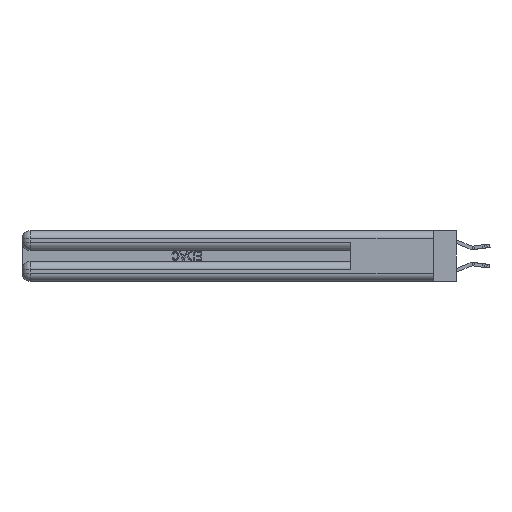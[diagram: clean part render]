
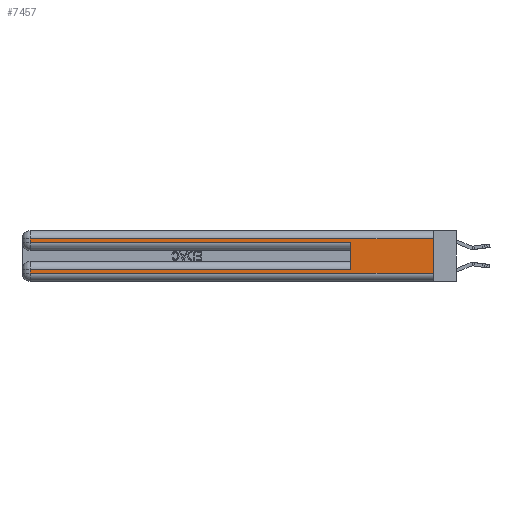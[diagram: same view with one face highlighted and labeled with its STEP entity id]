
A CAD part, left-side view. The second image highlights one B-rep face of the part: STEP entity #7457.
In plain terms, the highlighted planar face has unit normal (-1, 0, 0).
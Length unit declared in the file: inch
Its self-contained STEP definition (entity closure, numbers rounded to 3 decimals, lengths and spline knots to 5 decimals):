
#335 = CARTESIAN_POINT ( 'NONE',  ( 0., 0., 0.285 ) ) ;
#734 = VECTOR ( 'NONE', #7939, 39.37008 ) ;
#883 = DIRECTION ( 'NONE',  ( 0., 0., -1. ) ) ;
#1002 = LINE ( 'NONE', #26193, #14297 ) ;
#1200 = VERTEX_POINT ( 'NONE', #1347 ) ;
#1347 = CARTESIAN_POINT ( 'NONE',  ( 0., 0.6, 0.085 ) ) ;
#1394 = LINE ( 'NONE', #22031, #15465 ) ;
#2691 = DIRECTION ( 'NONE',  ( 0., 0., -1. ) ) ;
#3408 = EDGE_CURVE ( 'NONE', #15982, #7202, #14040, .T. ) ;
#3875 = ORIENTED_EDGE ( 'NONE', *, *, #21778, .F. ) ;
#4414 = DIRECTION ( 'NONE',  ( 0., 0., 1. ) ) ;
#6218 = LINE ( 'NONE', #8365, #31649 ) ;
#6445 = EDGE_LOOP ( 'NONE', ( #7116, #11155, #25132, #29296, #3875, #6481, #21207, #7955 ) ) ;
#6481 = ORIENTED_EDGE ( 'NONE', *, *, #14183, .T. ) ;
#7116 = ORIENTED_EDGE ( 'NONE', *, *, #29628, .F. ) ;
#7202 = VERTEX_POINT ( 'NONE', #16765 ) ;
#7212 = VERTEX_POINT ( 'NONE', #21712 ) ;
#7232 = DIRECTION ( 'NONE',  ( 0., -1., 0. ) ) ;
#7457 = ADVANCED_FACE ( 'NONE', ( #20144 ), #10488, .F. ) ;
#7765 = CARTESIAN_POINT ( 'NONE',  ( 0., 0., 0.37 ) ) ;
#7939 = DIRECTION ( 'NONE',  ( 0., -1., 0. ) ) ;
#7955 = ORIENTED_EDGE ( 'NONE', *, *, #30995, .T. ) ;
#8251 = DIRECTION ( 'NONE',  ( 0., 0., -1. ) ) ;
#8365 = CARTESIAN_POINT ( 'NONE',  ( 0., 2.94, 0.37 ) ) ;
#10486 = AXIS2_PLACEMENT_3D ( 'NONE', #7765, #27724, #13004 ) ;
#10488 = PLANE ( 'NONE',  #10486 ) ;
#11072 = LINE ( 'NONE', #19274, #29135 ) ;
#11155 = ORIENTED_EDGE ( 'NONE', *, *, #20409, .T. ) ;
#11357 = VERTEX_POINT ( 'NONE', #28933 ) ;
#12181 = CARTESIAN_POINT ( 'NONE',  ( 0., 0., 0.31 ) ) ;
#12823 = EDGE_CURVE ( 'NONE', #7212, #15982, #6218, .T. ) ;
#12826 = EDGE_CURVE ( 'NONE', #23387, #25735, #18623, .T. ) ;
#13004 = DIRECTION ( 'NONE',  ( 0., 0., -1. ) ) ;
#13632 = VECTOR ( 'NONE', #883, 39.37008 ) ;
#14040 = LINE ( 'NONE', #335, #734 ) ;
#14183 = EDGE_CURVE ( 'NONE', #1200, #23387, #1002, .T. ) ;
#14297 = VECTOR ( 'NONE', #28652, 39.37008 ) ;
#14634 = DIRECTION ( 'NONE',  ( 0., 1., 0. ) ) ;
#15465 = VECTOR ( 'NONE', #7232, 39.37008 ) ;
#15982 = VERTEX_POINT ( 'NONE', #17022 ) ;
#16765 = CARTESIAN_POINT ( 'NONE',  ( 0., 0.6, 0.285 ) ) ;
#17022 = CARTESIAN_POINT ( 'NONE',  ( 0., 2.94, 0.285 ) ) ;
#18623 = LINE ( 'NONE', #30545, #13632 ) ;
#19274 = CARTESIAN_POINT ( 'NONE',  ( 0., 0.6, 0.145 ) ) ;
#20144 = FACE_OUTER_BOUND ( 'NONE', #6445, .T. ) ;
#20409 = EDGE_CURVE ( 'NONE', #11357, #7212, #27702, .T. ) ;
#20541 = LINE ( 'NONE', #22554, #26314 ) ;
#20836 = CARTESIAN_POINT ( 'NONE',  ( 0., 0., 0.06 ) ) ;
#21017 = CARTESIAN_POINT ( 'NONE',  ( 0., 2.94, 0.085 ) ) ;
#21207 = ORIENTED_EDGE ( 'NONE', *, *, #12826, .T. ) ;
#21712 = CARTESIAN_POINT ( 'NONE',  ( 0., 2.94, 0.31 ) ) ;
#21778 = EDGE_CURVE ( 'NONE', #1200, #7202, #11072, .T. ) ;
#21930 = VECTOR ( 'NONE', #14634, 39.37008 ) ;
#22031 = CARTESIAN_POINT ( 'NONE',  ( 0., 0., 0.06 ) ) ;
#22554 = CARTESIAN_POINT ( 'NONE',  ( 0., 0., 0.37 ) ) ;
#22646 = VERTEX_POINT ( 'NONE', #20836 ) ;
#23387 = VERTEX_POINT ( 'NONE', #21017 ) ;
#25132 = ORIENTED_EDGE ( 'NONE', *, *, #12823, .T. ) ;
#25569 = CARTESIAN_POINT ( 'NONE',  ( 0., 2.94, 0.06 ) ) ;
#25735 = VERTEX_POINT ( 'NONE', #25569 ) ;
#26193 = CARTESIAN_POINT ( 'NONE',  ( 0., 0., 0.085 ) ) ;
#26314 = VECTOR ( 'NONE', #2691, 39.37008 ) ;
#27702 = LINE ( 'NONE', #12181, #21930 ) ;
#27724 = DIRECTION ( 'NONE',  ( 1., 0., 0. ) ) ;
#28652 = DIRECTION ( 'NONE',  ( 0., 1., 0. ) ) ;
#28933 = CARTESIAN_POINT ( 'NONE',  ( 0., 0., 0.31 ) ) ;
#29135 = VECTOR ( 'NONE', #4414, 39.37008 ) ;
#29296 = ORIENTED_EDGE ( 'NONE', *, *, #3408, .T. ) ;
#29628 = EDGE_CURVE ( 'NONE', #11357, #22646, #20541, .T. ) ;
#30545 = CARTESIAN_POINT ( 'NONE',  ( 0., 2.94, 0.37 ) ) ;
#30995 = EDGE_CURVE ( 'NONE', #25735, #22646, #1394, .T. ) ;
#31649 = VECTOR ( 'NONE', #8251, 39.37008 ) ;
